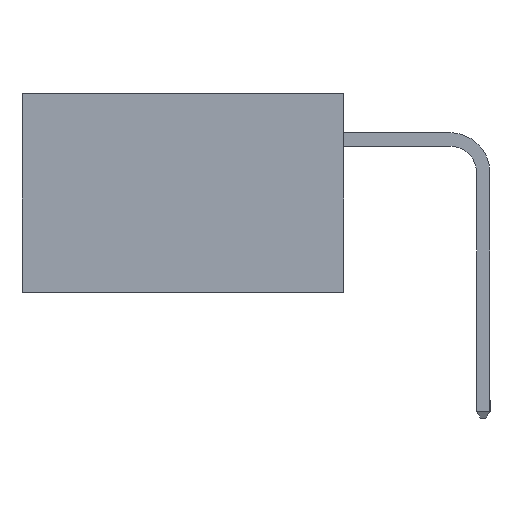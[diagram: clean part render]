
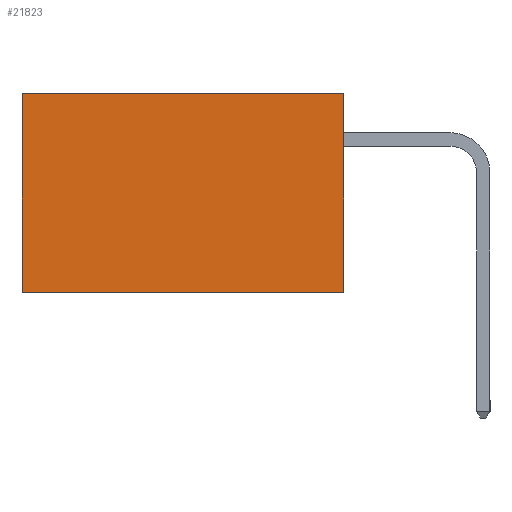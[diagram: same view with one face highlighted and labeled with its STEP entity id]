
A CAD part, left-side view. The second image highlights one B-rep face of the part: STEP entity #21823.
In plain terms, the highlighted planar face has unit normal (-1, 0, 0).
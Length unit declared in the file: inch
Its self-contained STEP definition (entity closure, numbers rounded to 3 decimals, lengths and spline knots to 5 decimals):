
#1336 = ORIENTED_EDGE ( 'NONE', *, *, #8187, .T. ) ;
#1897 = EDGE_CURVE ( 'NONE', #14993, #4192, #13584, .T. ) ;
#3196 = AXIS2_PLACEMENT_3D ( 'NONE', #17314, #19238, #7549 ) ;
#3227 = ORIENTED_EDGE ( 'NONE', *, *, #1897, .F. ) ;
#3284 = DIRECTION ( 'NONE',  ( 0., 0., -1. ) ) ;
#3308 = CARTESIAN_POINT ( 'NONE',  ( 0.2615, 0.6, -0.37 ) ) ;
#3351 = VECTOR ( 'NONE', #4344, 39.37008 ) ;
#3653 = PLANE ( 'NONE',  #3196 ) ;
#4046 = CARTESIAN_POINT ( 'NONE',  ( 0.2615, 0., 0. ) ) ;
#4192 = VERTEX_POINT ( 'NONE', #7656 ) ;
#4344 = DIRECTION ( 'NONE',  ( 0., 1., 0. ) ) ;
#7549 = DIRECTION ( 'NONE',  ( 0., 0., -1. ) ) ;
#7656 = CARTESIAN_POINT ( 'NONE',  ( 0.2615, 0.6, -0.37 ) ) ;
#8187 = EDGE_CURVE ( 'NONE', #15061, #4192, #20462, .T. ) ;
#8907 = EDGE_CURVE ( 'NONE', #24025, #15061, #9148, .T. ) ;
#9148 = LINE ( 'NONE', #4046, #3351 ) ;
#9622 = CARTESIAN_POINT ( 'NONE',  ( 0.2615, 0., -0.37 ) ) ;
#10100 = VECTOR ( 'NONE', #3284, 39.37008 ) ;
#10707 = CARTESIAN_POINT ( 'NONE',  ( 0.2615, 0., 0. ) ) ;
#11613 = DIRECTION ( 'NONE',  ( 0., 0., -1. ) ) ;
#12015 = EDGE_LOOP ( 'NONE', ( #1336, #3227, #21021, #14630 ) ) ;
#13584 = LINE ( 'NONE', #24292, #18121 ) ;
#14630 = ORIENTED_EDGE ( 'NONE', *, *, #8907, .T. ) ;
#14993 = VERTEX_POINT ( 'NONE', #19694 ) ;
#15061 = VERTEX_POINT ( 'NONE', #18110 ) ;
#15502 = EDGE_CURVE ( 'NONE', #24025, #14993, #24967, .T. ) ;
#17314 = CARTESIAN_POINT ( 'NONE',  ( 0.2615, 0., -0.37 ) ) ;
#18110 = CARTESIAN_POINT ( 'NONE',  ( 0.2615, 0.6, 0. ) ) ;
#18121 = VECTOR ( 'NONE', #20609, 39.37008 ) ;
#19238 = DIRECTION ( 'NONE',  ( 1., 0., 0. ) ) ;
#19694 = CARTESIAN_POINT ( 'NONE',  ( 0.2615, 0., -0.37 ) ) ;
#20462 = LINE ( 'NONE', #3308, #10100 ) ;
#20609 = DIRECTION ( 'NONE',  ( 0., 1., 0. ) ) ;
#21021 = ORIENTED_EDGE ( 'NONE', *, *, #15502, .F. ) ;
#21823 = ADVANCED_FACE ( 'NONE', ( #24715 ), #3653, .F. ) ;
#23837 = VECTOR ( 'NONE', #11613, 39.37008 ) ;
#24025 = VERTEX_POINT ( 'NONE', #10707 ) ;
#24292 = CARTESIAN_POINT ( 'NONE',  ( 0.2615, 0., -0.37 ) ) ;
#24715 = FACE_OUTER_BOUND ( 'NONE', #12015, .T. ) ;
#24967 = LINE ( 'NONE', #9622, #23837 ) ;
